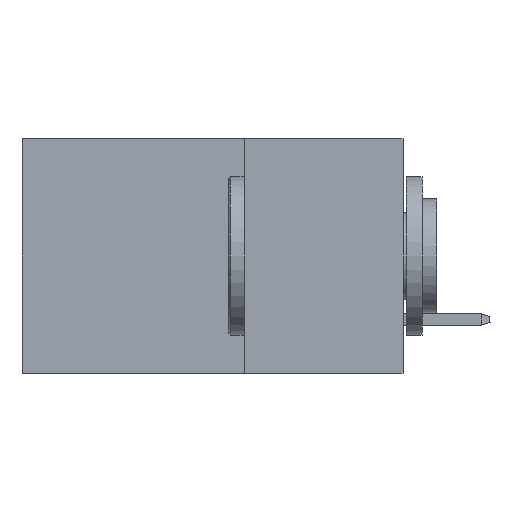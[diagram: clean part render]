
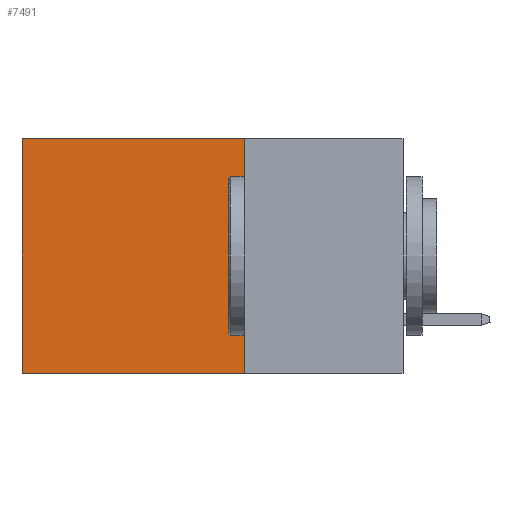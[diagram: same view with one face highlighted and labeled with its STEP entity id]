
A CAD part, left-side view. The second image highlights one B-rep face of the part: STEP entity #7491.
In plain terms, the highlighted planar face has unit normal (-1, 0, 0).
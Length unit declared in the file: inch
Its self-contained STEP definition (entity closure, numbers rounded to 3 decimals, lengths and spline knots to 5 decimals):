
#1739 = LINE ( 'NONE', #8263, #30403 ) ;
#4227 = CARTESIAN_POINT ( 'NONE',  ( 0.2875, 0.25, 0. ) ) ;
#4236 = DIRECTION ( 'NONE',  ( 0., 1., 0. ) ) ;
#5550 = ORIENTED_EDGE ( 'NONE', *, *, #19009, .F. ) ;
#6824 = FACE_OUTER_BOUND ( 'NONE', #9554, .T. ) ;
#7491 = ADVANCED_FACE ( 'NONE', ( #6824 ), #13106, .F. ) ;
#7543 = VECTOR ( 'NONE', #4236, 39.37008 ) ;
#8099 = VECTOR ( 'NONE', #18293, 39.37008 ) ;
#8263 = CARTESIAN_POINT ( 'NONE',  ( 0.2875, 0.6, 0. ) ) ;
#8330 = VECTOR ( 'NONE', #15771, 39.37008 ) ;
#9484 = LINE ( 'NONE', #24587, #8099 ) ;
#9554 = EDGE_LOOP ( 'NONE', ( #23021, #5550, #11926, #15192 ) ) ;
#11926 = ORIENTED_EDGE ( 'NONE', *, *, #28110, .F. ) ;
#12407 = VERTEX_POINT ( 'NONE', #34970 ) ;
#13106 = PLANE ( 'NONE',  #17104 ) ;
#13450 = CARTESIAN_POINT ( 'NONE',  ( 0.2875, 0.6, 0. ) ) ;
#15096 = EDGE_CURVE ( 'NONE', #17765, #31009, #9484, .T. ) ;
#15192 = ORIENTED_EDGE ( 'NONE', *, *, #15096, .T. ) ;
#15771 = DIRECTION ( 'NONE',  ( 0., 0., -1. ) ) ;
#16697 = CARTESIAN_POINT ( 'NONE',  ( 0.2875, 0.25, 0. ) ) ;
#17104 = AXIS2_PLACEMENT_3D ( 'NONE', #16697, #38580, #38790 ) ;
#17765 = VERTEX_POINT ( 'NONE', #4227 ) ;
#18293 = DIRECTION ( 'NONE',  ( 0., 1., 0. ) ) ;
#19009 = EDGE_CURVE ( 'NONE', #12407, #35993, #39356, .T. ) ;
#19853 = EDGE_CURVE ( 'NONE', #31009, #35993, #1739, .T. ) ;
#20629 = DIRECTION ( 'NONE',  ( 0., 0., -1. ) ) ;
#23021 = ORIENTED_EDGE ( 'NONE', *, *, #19853, .T. ) ;
#23883 = CARTESIAN_POINT ( 'NONE',  ( 0.2875, 0.6, -0.37 ) ) ;
#24587 = CARTESIAN_POINT ( 'NONE',  ( 0.2875, 0.25, 0. ) ) ;
#25227 = LINE ( 'NONE', #31751, #8330 ) ;
#28110 = EDGE_CURVE ( 'NONE', #17765, #12407, #25227, .T. ) ;
#30403 = VECTOR ( 'NONE', #20629, 39.37008 ) ;
#31009 = VERTEX_POINT ( 'NONE', #13450 ) ;
#31751 = CARTESIAN_POINT ( 'NONE',  ( 0.2875, 0.25, 0. ) ) ;
#34970 = CARTESIAN_POINT ( 'NONE',  ( 0.2875, 0.25, -0.37 ) ) ;
#35993 = VERTEX_POINT ( 'NONE', #23883 ) ;
#36399 = CARTESIAN_POINT ( 'NONE',  ( 0.2875, 0.25, -0.37 ) ) ;
#38580 = DIRECTION ( 'NONE',  ( 1., 0., 0. ) ) ;
#38790 = DIRECTION ( 'NONE',  ( 0., 0., -1. ) ) ;
#39356 = LINE ( 'NONE', #36399, #7543 ) ;
